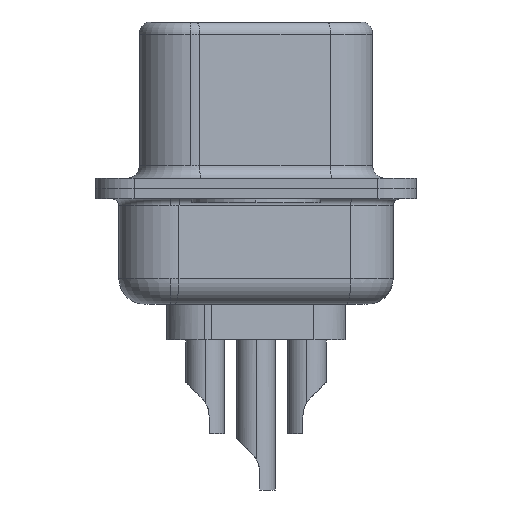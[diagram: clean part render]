
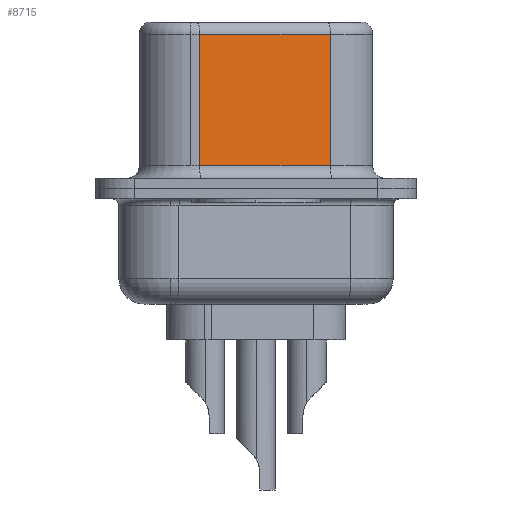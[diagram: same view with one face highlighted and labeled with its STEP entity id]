
A CAD part, left-side view. The second image highlights one B-rep face of the part: STEP entity #8715.
In plain terms, the highlighted planar face has unit normal (-0.985, -0.174, 0).
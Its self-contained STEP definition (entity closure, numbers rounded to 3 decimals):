
#333 = CARTESIAN_POINT ( 'NONE',  ( 4.58, -2.897, 0.9 ) ) ;
#1059 = DIRECTION ( 'NONE',  ( -0.174, 0.985, 0. ) ) ;
#1127 = LINE ( 'NONE', #20438, #15956 ) ;
#1329 = DIRECTION ( 'NONE',  ( 0.174, -0.985, 0. ) ) ;
#1694 = VERTEX_POINT ( 'NONE', #17684 ) ;
#2242 = VECTOR ( 'NONE', #1329, 1000. ) ;
#2287 = ORIENTED_EDGE ( 'NONE', *, *, #4620, .T. ) ;
#2865 = LINE ( 'NONE', #15627, #2242 ) ;
#3688 = FACE_OUTER_BOUND ( 'NONE', #9643, .T. ) ;
#4620 = EDGE_CURVE ( 'NONE', #1694, #23048, #10807, .T. ) ;
#5016 = DIRECTION ( 'NONE',  ( -0.174, 0.985, 0. ) ) ;
#5231 = LINE ( 'NONE', #24742, #13745 ) ;
#6106 = EDGE_CURVE ( 'NONE', #9980, #22679, #2865, .T. ) ;
#8715 = ADVANCED_FACE ( 'NONE', ( #3688 ), #24099, .F. ) ;
#8941 = CARTESIAN_POINT ( 'NONE',  ( 3.68, 2.203, 0.9 ) ) ;
#9643 = EDGE_LOOP ( 'NONE', ( #24076, #2287, #18891, #15036 ) ) ;
#9980 = VERTEX_POINT ( 'NONE', #8941 ) ;
#9990 = CARTESIAN_POINT ( 'NONE',  ( 4.58, -2.897, 6.02 ) ) ;
#10734 = CARTESIAN_POINT ( 'NONE',  ( 4.58, -2.897, 6.52 ) ) ;
#10807 = LINE ( 'NONE', #9990, #24840 ) ;
#11313 = DIRECTION ( 'NONE',  ( 0., 0., -1. ) ) ;
#12697 = DIRECTION ( 'NONE',  ( 0.985, 0.174, 0. ) ) ;
#13745 = VECTOR ( 'NONE', #11313, 1000. ) ;
#14688 = DIRECTION ( 'NONE',  ( 0., 0., -1. ) ) ;
#15036 = ORIENTED_EDGE ( 'NONE', *, *, #6106, .T. ) ;
#15627 = CARTESIAN_POINT ( 'NONE',  ( 4.58, -2.897, 0.9 ) ) ;
#15956 = VECTOR ( 'NONE', #14688, 1000. ) ;
#17684 = CARTESIAN_POINT ( 'NONE',  ( 4.58, -2.897, 6.02 ) ) ;
#17965 = EDGE_CURVE ( 'NONE', #23048, #9980, #1127, .T. ) ;
#18829 = CARTESIAN_POINT ( 'NONE',  ( 3.68, 2.203, 6.02 ) ) ;
#18891 = ORIENTED_EDGE ( 'NONE', *, *, #17965, .T. ) ;
#20438 = CARTESIAN_POINT ( 'NONE',  ( 3.68, 2.203, 6.52 ) ) ;
#22081 = EDGE_CURVE ( 'NONE', #1694, #22679, #5231, .T. ) ;
#22679 = VERTEX_POINT ( 'NONE', #333 ) ;
#23048 = VERTEX_POINT ( 'NONE', #18829 ) ;
#23068 = AXIS2_PLACEMENT_3D ( 'NONE', #10734, #12697, #1059 ) ;
#24076 = ORIENTED_EDGE ( 'NONE', *, *, #22081, .F. ) ;
#24099 = PLANE ( 'NONE',  #23068 ) ;
#24742 = CARTESIAN_POINT ( 'NONE',  ( 4.58, -2.897, 6.52 ) ) ;
#24840 = VECTOR ( 'NONE', #5016, 1000. ) ;
